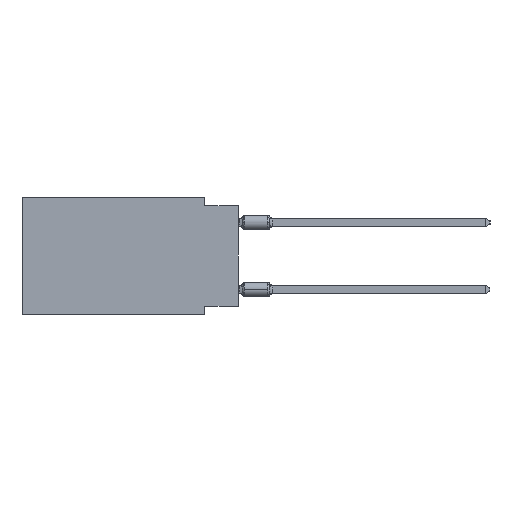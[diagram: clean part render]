
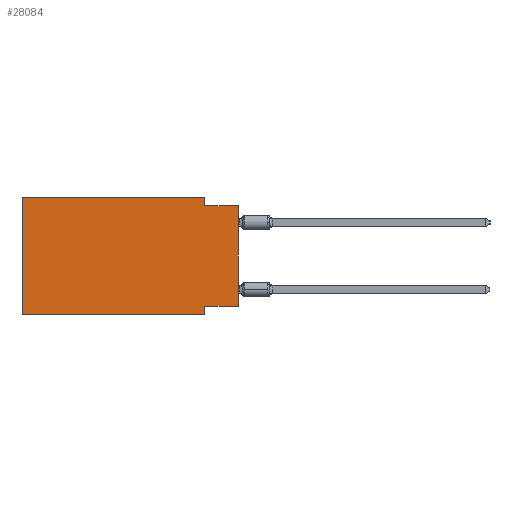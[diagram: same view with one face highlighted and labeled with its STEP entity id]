
A CAD part, left-side view. The second image highlights one B-rep face of the part: STEP entity #28084.
In plain terms, the highlighted planar face has unit normal (-1, 0, 0).
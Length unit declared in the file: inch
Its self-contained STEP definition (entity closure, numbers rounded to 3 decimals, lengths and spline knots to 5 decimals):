
#55 = CARTESIAN_POINT ( 'NONE',  ( 0., 0.1, 0. ) ) ;
#355 = DIRECTION ( 'NONE',  ( 0., 0., 1. ) ) ;
#457 = ORIENTED_EDGE ( 'NONE', *, *, #38439, .F. ) ;
#868 = VECTOR ( 'NONE', #355, 39.37008 ) ;
#1948 = LINE ( 'NONE', #33268, #4020 ) ;
#2379 = EDGE_CURVE ( 'NONE', #26083, #27059, #30806, .T. ) ;
#2659 = VERTEX_POINT ( 'NONE', #25765 ) ;
#4020 = VECTOR ( 'NONE', #4822, 39.37008 ) ;
#4265 = ORIENTED_EDGE ( 'NONE', *, *, #27163, .F. ) ;
#4822 = DIRECTION ( 'NONE',  ( 0., 1., 0. ) ) ;
#5389 = EDGE_CURVE ( 'NONE', #29298, #2659, #22292, .T. ) ;
#6370 = EDGE_CURVE ( 'NONE', #29298, #18332, #8530, .T. ) ;
#6982 = DIRECTION ( 'NONE',  ( 0., 0., 1. ) ) ;
#7530 = VECTOR ( 'NONE', #38766, 39.37008 ) ;
#7665 = CARTESIAN_POINT ( 'NONE',  ( 0., 0., -0.325 ) ) ;
#8213 = VERTEX_POINT ( 'NONE', #18869 ) ;
#8530 = LINE ( 'NONE', #27575, #10646 ) ;
#8993 = CARTESIAN_POINT ( 'NONE',  ( 0., 0.645, 0. ) ) ;
#10032 = ORIENTED_EDGE ( 'NONE', *, *, #6370, .T. ) ;
#10256 = PLANE ( 'NONE',  #32067 ) ;
#10597 = CARTESIAN_POINT ( 'NONE',  ( 0., 0.1, -0.35 ) ) ;
#10646 = VECTOR ( 'NONE', #24527, 39.37008 ) ;
#13021 = VECTOR ( 'NONE', #6982, 39.37008 ) ;
#13332 = CARTESIAN_POINT ( 'NONE',  ( 0., 0.645, 0. ) ) ;
#13471 = EDGE_CURVE ( 'NONE', #8213, #18332, #29409, .T. ) ;
#13524 = ORIENTED_EDGE ( 'NONE', *, *, #17930, .F. ) ;
#15552 = CARTESIAN_POINT ( 'NONE',  ( 0., 0.645, 0. ) ) ;
#16106 = CARTESIAN_POINT ( 'NONE',  ( 0., 0., -0.025 ) ) ;
#16654 = VERTEX_POINT ( 'NONE', #16106 ) ;
#17668 = VECTOR ( 'NONE', #25448, 39.37008 ) ;
#17789 = ORIENTED_EDGE ( 'NONE', *, *, #26843, .T. ) ;
#17899 = VECTOR ( 'NONE', #38825, 39.37008 ) ;
#17930 = EDGE_CURVE ( 'NONE', #23120, #8213, #1948, .T. ) ;
#18041 = LINE ( 'NONE', #8993, #22902 ) ;
#18332 = VERTEX_POINT ( 'NONE', #10597 ) ;
#18869 = CARTESIAN_POINT ( 'NONE',  ( 0., 0.1, -0.325 ) ) ;
#19479 = DIRECTION ( 'NONE',  ( 0., 0., -1. ) ) ;
#20923 = CARTESIAN_POINT ( 'NONE',  ( 0., 0.1, 0. ) ) ;
#21520 = CARTESIAN_POINT ( 'NONE',  ( 0., 0.1, -0.025 ) ) ;
#22292 = LINE ( 'NONE', #15552, #868 ) ;
#22902 = VECTOR ( 'NONE', #33974, 39.37008 ) ;
#23120 = VERTEX_POINT ( 'NONE', #7665 ) ;
#23138 = ORIENTED_EDGE ( 'NONE', *, *, #2379, .F. ) ;
#24527 = DIRECTION ( 'NONE',  ( 0., -1., 0. ) ) ;
#25448 = DIRECTION ( 'NONE',  ( 0., 0., -1. ) ) ;
#25596 = FACE_OUTER_BOUND ( 'NONE', #29471, .T. ) ;
#25765 = CARTESIAN_POINT ( 'NONE',  ( 0., 0.645, 0. ) ) ;
#26076 = LINE ( 'NONE', #34892, #7530 ) ;
#26083 = VERTEX_POINT ( 'NONE', #20923 ) ;
#26346 = CARTESIAN_POINT ( 'NONE',  ( 0., 0.1, -0.35 ) ) ;
#26843 = EDGE_CURVE ( 'NONE', #23120, #16654, #29082, .T. ) ;
#27059 = VERTEX_POINT ( 'NONE', #21520 ) ;
#27163 = EDGE_CURVE ( 'NONE', #2659, #26083, #18041, .T. ) ;
#27575 = CARTESIAN_POINT ( 'NONE',  ( 0., 0.645, -0.35 ) ) ;
#28084 = ADVANCED_FACE ( 'NONE', ( #25596 ), #10256, .F. ) ;
#29082 = LINE ( 'NONE', #34616, #13021 ) ;
#29298 = VERTEX_POINT ( 'NONE', #38489 ) ;
#29409 = LINE ( 'NONE', #26346, #17899 ) ;
#29471 = EDGE_LOOP ( 'NONE', ( #17789, #457, #23138, #4265, #36435, #10032, #34513, #13524 ) ) ;
#30806 = LINE ( 'NONE', #55, #17668 ) ;
#32067 = AXIS2_PLACEMENT_3D ( 'NONE', #13332, #35045, #19479 ) ;
#33268 = CARTESIAN_POINT ( 'NONE',  ( 0., 0., -0.325 ) ) ;
#33974 = DIRECTION ( 'NONE',  ( 0., -1., 0. ) ) ;
#34513 = ORIENTED_EDGE ( 'NONE', *, *, #13471, .F. ) ;
#34616 = CARTESIAN_POINT ( 'NONE',  ( 0., 0., 0. ) ) ;
#34892 = CARTESIAN_POINT ( 'NONE',  ( 0., 0., -0.025 ) ) ;
#35045 = DIRECTION ( 'NONE',  ( 1., 0., 0. ) ) ;
#36435 = ORIENTED_EDGE ( 'NONE', *, *, #5389, .F. ) ;
#38439 = EDGE_CURVE ( 'NONE', #27059, #16654, #26076, .T. ) ;
#38489 = CARTESIAN_POINT ( 'NONE',  ( 0., 0.645, -0.35 ) ) ;
#38766 = DIRECTION ( 'NONE',  ( 0., -1., 0. ) ) ;
#38825 = DIRECTION ( 'NONE',  ( 0., 0., -1. ) ) ;
